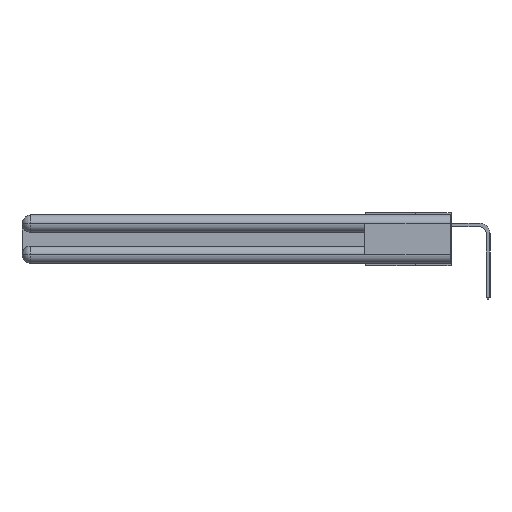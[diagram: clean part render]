
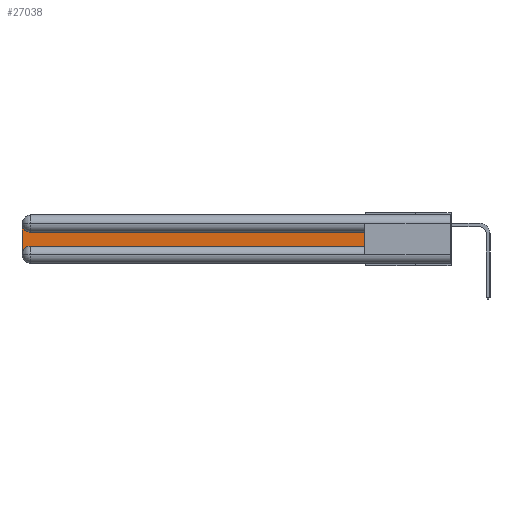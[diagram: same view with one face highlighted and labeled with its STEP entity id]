
A CAD part, left-side view. The second image highlights one B-rep face of the part: STEP entity #27038.
In plain terms, the highlighted planar face has unit normal (-1, 0, 0).
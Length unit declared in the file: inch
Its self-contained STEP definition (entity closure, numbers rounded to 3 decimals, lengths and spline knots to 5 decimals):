
#741 = CARTESIAN_POINT ( 'NONE',  ( 0.075, 0.6, -0.2175 ) ) ;
#775 = ORIENTED_EDGE ( 'NONE', *, *, #8543, .T. ) ;
#912 = CARTESIAN_POINT ( 'NONE',  ( 0.075, 0.6, -0.2175 ) ) ;
#1022 = DIRECTION ( 'NONE',  ( 0., 0., 1. ) ) ;
#1393 = VERTEX_POINT ( 'NONE', #10242 ) ;
#1692 = DIRECTION ( 'NONE',  ( 0., 0., -1. ) ) ;
#2206 = LINE ( 'NONE', #16830, #12718 ) ;
#2585 = LINE ( 'NONE', #18857, #16250 ) ;
#3988 = CARTESIAN_POINT ( 'NONE',  ( 0.075, 0.6, -0.1225 ) ) ;
#4750 = VERTEX_POINT ( 'NONE', #741 ) ;
#4997 = CARTESIAN_POINT ( 'NONE',  ( 0.075, 3., -0.0625 ) ) ;
#5285 = EDGE_LOOP ( 'NONE', ( #28390, #11892, #26732, #775, #17506, #19890 ) ) ;
#6578 = DIRECTION ( 'NONE',  ( 0., 0., -1. ) ) ;
#6779 = LINE ( 'NONE', #912, #23185 ) ;
#6784 = CIRCLE ( 'NONE', #28275, 0.06 ) ;
#6840 = DIRECTION ( 'NONE',  ( 0., 0., -1. ) ) ;
#6904 = CIRCLE ( 'NONE', #20516, 0.06 ) ;
#7146 = EDGE_CURVE ( 'NONE', #14981, #1393, #13314, .T. ) ;
#8543 = EDGE_CURVE ( 'NONE', #25538, #27087, #6904, .T. ) ;
#8861 = CARTESIAN_POINT ( 'NONE',  ( 0.075, 2.94, -0.0625 ) ) ;
#10242 = CARTESIAN_POINT ( 'NONE',  ( 0.075, 2.94, -0.1225 ) ) ;
#10883 = CARTESIAN_POINT ( 'NONE',  ( 0.075, 2.94, -0.2775 ) ) ;
#11357 = EDGE_CURVE ( 'NONE', #4750, #14981, #6779, .T. ) ;
#11490 = FACE_OUTER_BOUND ( 'NONE', #5285, .T. ) ;
#11892 = ORIENTED_EDGE ( 'NONE', *, *, #13270, .T. ) ;
#12120 = VERTEX_POINT ( 'NONE', #4997 ) ;
#12123 = CARTESIAN_POINT ( 'NONE',  ( 0.075, 3., -0.2775 ) ) ;
#12525 = EDGE_CURVE ( 'NONE', #27087, #4750, #2585, .T. ) ;
#12718 = VECTOR ( 'NONE', #6840, 39.37008 ) ;
#13270 = EDGE_CURVE ( 'NONE', #1393, #12120, #6784, .T. ) ;
#13314 = LINE ( 'NONE', #27093, #26258 ) ;
#13557 = DIRECTION ( 'NONE',  ( 0., 0., -1. ) ) ;
#14165 = EDGE_CURVE ( 'NONE', #12120, #25538, #2206, .T. ) ;
#14981 = VERTEX_POINT ( 'NONE', #3988 ) ;
#15579 = DIRECTION ( 'NONE',  ( 1., 0., 0. ) ) ;
#16250 = VECTOR ( 'NONE', #16585, 39.37008 ) ;
#16585 = DIRECTION ( 'NONE',  ( 0., -1., 0. ) ) ;
#16830 = CARTESIAN_POINT ( 'NONE',  ( 0.075, 3., -0.2175 ) ) ;
#17363 = DIRECTION ( 'NONE',  ( 1., 0., 0. ) ) ;
#17506 = ORIENTED_EDGE ( 'NONE', *, *, #12525, .T. ) ;
#18857 = CARTESIAN_POINT ( 'NONE',  ( 0.075, 0.6, -0.2175 ) ) ;
#19723 = CARTESIAN_POINT ( 'NONE',  ( 0.075, 3., -0.1225 ) ) ;
#19890 = ORIENTED_EDGE ( 'NONE', *, *, #11357, .T. ) ;
#20516 = AXIS2_PLACEMENT_3D ( 'NONE', #10883, #15579, #6578 ) ;
#20974 = AXIS2_PLACEMENT_3D ( 'NONE', #19723, #17363, #1692 ) ;
#23185 = VECTOR ( 'NONE', #1022, 39.37008 ) ;
#23628 = CARTESIAN_POINT ( 'NONE',  ( 0.075, 2.94, -0.2175 ) ) ;
#24708 = DIRECTION ( 'NONE',  ( 1., 0., 0. ) ) ;
#24943 = DIRECTION ( 'NONE',  ( 0., 1., 0. ) ) ;
#25538 = VERTEX_POINT ( 'NONE', #12123 ) ;
#26258 = VECTOR ( 'NONE', #24943, 39.37008 ) ;
#26732 = ORIENTED_EDGE ( 'NONE', *, *, #14165, .T. ) ;
#27038 = ADVANCED_FACE ( 'NONE', ( #11490 ), #28731, .F. ) ;
#27087 = VERTEX_POINT ( 'NONE', #23628 ) ;
#27093 = CARTESIAN_POINT ( 'NONE',  ( 0.075, 0.6, -0.1225 ) ) ;
#28275 = AXIS2_PLACEMENT_3D ( 'NONE', #8861, #24708, #13557 ) ;
#28390 = ORIENTED_EDGE ( 'NONE', *, *, #7146, .T. ) ;
#28731 = PLANE ( 'NONE',  #20974 ) ;
